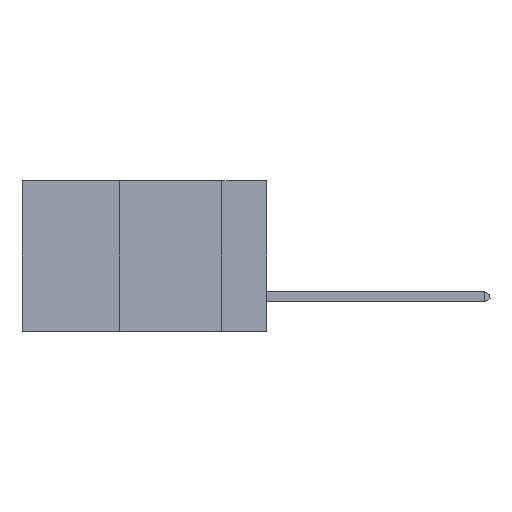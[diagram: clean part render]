
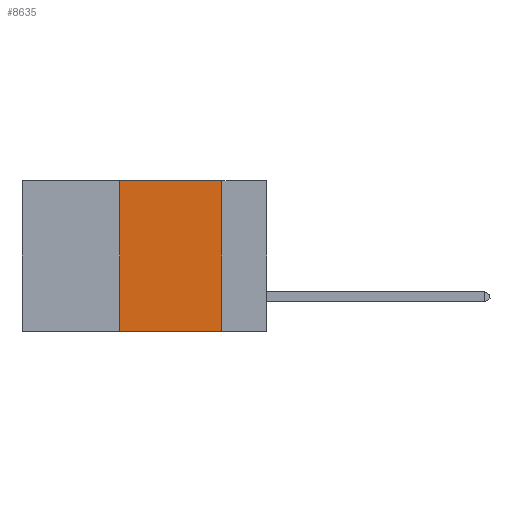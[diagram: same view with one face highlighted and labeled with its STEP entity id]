
A CAD part, left-side view. The second image highlights one B-rep face of the part: STEP entity #8635.
In plain terms, the highlighted planar face has unit normal (-1, 0, 0).
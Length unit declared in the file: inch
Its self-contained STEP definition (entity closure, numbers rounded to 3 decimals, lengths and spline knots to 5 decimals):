
#637 = CARTESIAN_POINT ( 'NONE',  ( 0., 0.6, 0. ) ) ;
#1108 = VECTOR ( 'NONE', #2879, 39.37008 ) ;
#1457 = EDGE_CURVE ( 'NONE', #6735, #13783, #16176, .T. ) ;
#1580 = LINE ( 'NONE', #11784, #13012 ) ;
#1666 = AXIS2_PLACEMENT_3D ( 'NONE', #637, #2203, #12628 ) ;
#2203 = DIRECTION ( 'NONE',  ( 1., 0., 0. ) ) ;
#2253 = LINE ( 'NONE', #10030, #9385 ) ;
#2572 = EDGE_CURVE ( 'NONE', #4114, #11741, #2253, .T. ) ;
#2586 = ORIENTED_EDGE ( 'NONE', *, *, #1457, .F. ) ;
#2879 = DIRECTION ( 'NONE',  ( 0., -1., 0. ) ) ;
#3692 = FACE_OUTER_BOUND ( 'NONE', #17256, .T. ) ;
#3754 = LINE ( 'NONE', #17315, #11299 ) ;
#4114 = VERTEX_POINT ( 'NONE', #13183 ) ;
#4932 = ORIENTED_EDGE ( 'NONE', *, *, #2572, .T. ) ;
#6677 = PLANE ( 'NONE',  #1666 ) ;
#6735 = VERTEX_POINT ( 'NONE', #7602 ) ;
#7602 = CARTESIAN_POINT ( 'NONE',  ( 0., 0.36, 0. ) ) ;
#8598 = CARTESIAN_POINT ( 'NONE',  ( 0., 0.11, -0.37 ) ) ;
#8635 = ADVANCED_FACE ( 'NONE', ( #3692 ), #6677, .F. ) ;
#9385 = VECTOR ( 'NONE', #10108, 39.37008 ) ;
#10030 = CARTESIAN_POINT ( 'NONE',  ( 0., 0.6, -0.37 ) ) ;
#10108 = DIRECTION ( 'NONE',  ( 0., -1., 0. ) ) ;
#11299 = VECTOR ( 'NONE', #14642, 39.37008 ) ;
#11741 = VERTEX_POINT ( 'NONE', #8598 ) ;
#11784 = CARTESIAN_POINT ( 'NONE',  ( 0., 0.11, 0. ) ) ;
#11842 = DIRECTION ( 'NONE',  ( 0., 0., -1. ) ) ;
#12628 = DIRECTION ( 'NONE',  ( 0., 0., -1. ) ) ;
#13012 = VECTOR ( 'NONE', #11842, 39.37008 ) ;
#13054 = EDGE_CURVE ( 'NONE', #4114, #6735, #3754, .T. ) ;
#13183 = CARTESIAN_POINT ( 'NONE',  ( 0., 0.36, -0.37 ) ) ;
#13643 = EDGE_CURVE ( 'NONE', #13783, #11741, #1580, .T. ) ;
#13783 = VERTEX_POINT ( 'NONE', #16237 ) ;
#14642 = DIRECTION ( 'NONE',  ( 0., 0., 1. ) ) ;
#16176 = LINE ( 'NONE', #18548, #1108 ) ;
#16237 = CARTESIAN_POINT ( 'NONE',  ( 0., 0.11, 0. ) ) ;
#17035 = ORIENTED_EDGE ( 'NONE', *, *, #13643, .F. ) ;
#17256 = EDGE_LOOP ( 'NONE', ( #17035, #2586, #17273, #4932 ) ) ;
#17273 = ORIENTED_EDGE ( 'NONE', *, *, #13054, .F. ) ;
#17315 = CARTESIAN_POINT ( 'NONE',  ( 0., 0.36, 0. ) ) ;
#18548 = CARTESIAN_POINT ( 'NONE',  ( 0., 0.6, 0. ) ) ;
